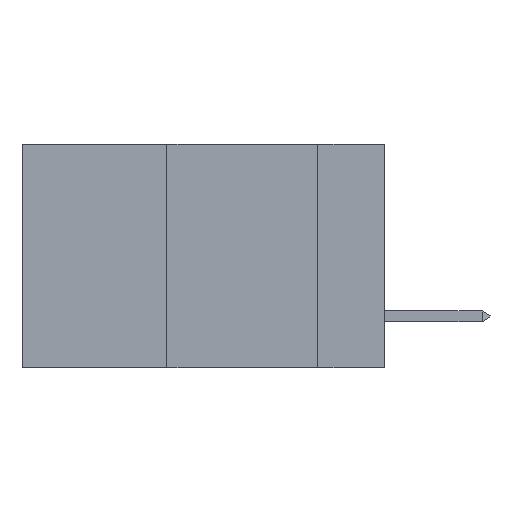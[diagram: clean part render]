
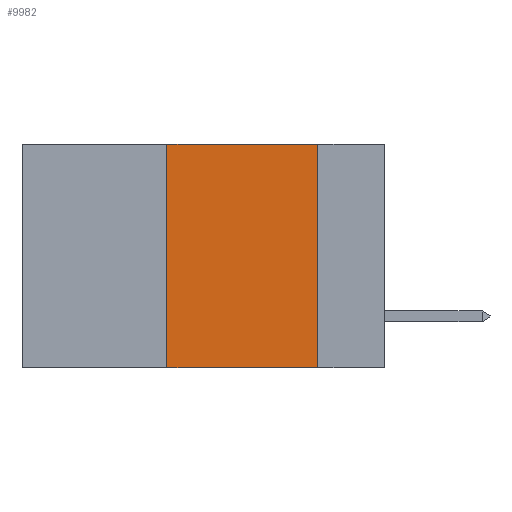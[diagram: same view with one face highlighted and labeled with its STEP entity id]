
A CAD part, left-side view. The second image highlights one B-rep face of the part: STEP entity #9982.
In plain terms, the highlighted planar face has unit normal (-1, 0, 0).
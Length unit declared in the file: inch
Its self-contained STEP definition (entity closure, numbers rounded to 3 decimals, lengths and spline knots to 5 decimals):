
#597 = EDGE_CURVE ( 'NONE', #3590, #6454, #15276, .T. ) ;
#659 = DIRECTION ( 'NONE',  ( 0., 0., -1. ) ) ;
#2131 = CARTESIAN_POINT ( 'NONE',  ( 0., 0.36, 0. ) ) ;
#3590 = VERTEX_POINT ( 'NONE', #21740 ) ;
#4562 = CARTESIAN_POINT ( 'NONE',  ( 0., 0.6, 0. ) ) ;
#5168 = VECTOR ( 'NONE', #17250, 39.37008 ) ;
#5253 = VERTEX_POINT ( 'NONE', #22999 ) ;
#5691 = CARTESIAN_POINT ( 'NONE',  ( 0., 0.36, -0.37 ) ) ;
#6430 = CARTESIAN_POINT ( 'NONE',  ( 0., 0.11, 0. ) ) ;
#6454 = VERTEX_POINT ( 'NONE', #14266 ) ;
#7035 = CARTESIAN_POINT ( 'NONE',  ( 0., 0.6, -0.37 ) ) ;
#7412 = PLANE ( 'NONE',  #19788 ) ;
#8324 = VERTEX_POINT ( 'NONE', #5691 ) ;
#9622 = ORIENTED_EDGE ( 'NONE', *, *, #18171, .F. ) ;
#9683 = ORIENTED_EDGE ( 'NONE', *, *, #597, .F. ) ;
#9808 = DIRECTION ( 'NONE',  ( 0., -1., 0. ) ) ;
#9982 = ADVANCED_FACE ( 'NONE', ( #14626 ), #7412, .F. ) ;
#11288 = VECTOR ( 'NONE', #14129, 39.37008 ) ;
#11524 = EDGE_CURVE ( 'NONE', #8324, #6454, #13911, .T. ) ;
#11891 = LINE ( 'NONE', #4562, #16512 ) ;
#12475 = EDGE_LOOP ( 'NONE', ( #9683, #20262, #9622, #21835 ) ) ;
#12948 = LINE ( 'NONE', #2131, #18386 ) ;
#13478 = EDGE_CURVE ( 'NONE', #5253, #3590, #11891, .T. ) ;
#13911 = LINE ( 'NONE', #7035, #11288 ) ;
#14129 = DIRECTION ( 'NONE',  ( 0., -1., 0. ) ) ;
#14266 = CARTESIAN_POINT ( 'NONE',  ( 0., 0.11, -0.37 ) ) ;
#14626 = FACE_OUTER_BOUND ( 'NONE', #12475, .T. ) ;
#15276 = LINE ( 'NONE', #6430, #5168 ) ;
#16512 = VECTOR ( 'NONE', #9808, 39.37008 ) ;
#16573 = DIRECTION ( 'NONE',  ( 0., 0., 1. ) ) ;
#17250 = DIRECTION ( 'NONE',  ( 0., 0., -1. ) ) ;
#18171 = EDGE_CURVE ( 'NONE', #8324, #5253, #12948, .T. ) ;
#18386 = VECTOR ( 'NONE', #16573, 39.37008 ) ;
#19638 = DIRECTION ( 'NONE',  ( 1., 0., 0. ) ) ;
#19753 = CARTESIAN_POINT ( 'NONE',  ( 0., 0.6, 0. ) ) ;
#19788 = AXIS2_PLACEMENT_3D ( 'NONE', #19753, #19638, #659 ) ;
#20262 = ORIENTED_EDGE ( 'NONE', *, *, #13478, .F. ) ;
#21740 = CARTESIAN_POINT ( 'NONE',  ( 0., 0.11, 0. ) ) ;
#21835 = ORIENTED_EDGE ( 'NONE', *, *, #11524, .T. ) ;
#22999 = CARTESIAN_POINT ( 'NONE',  ( 0., 0.36, 0. ) ) ;
